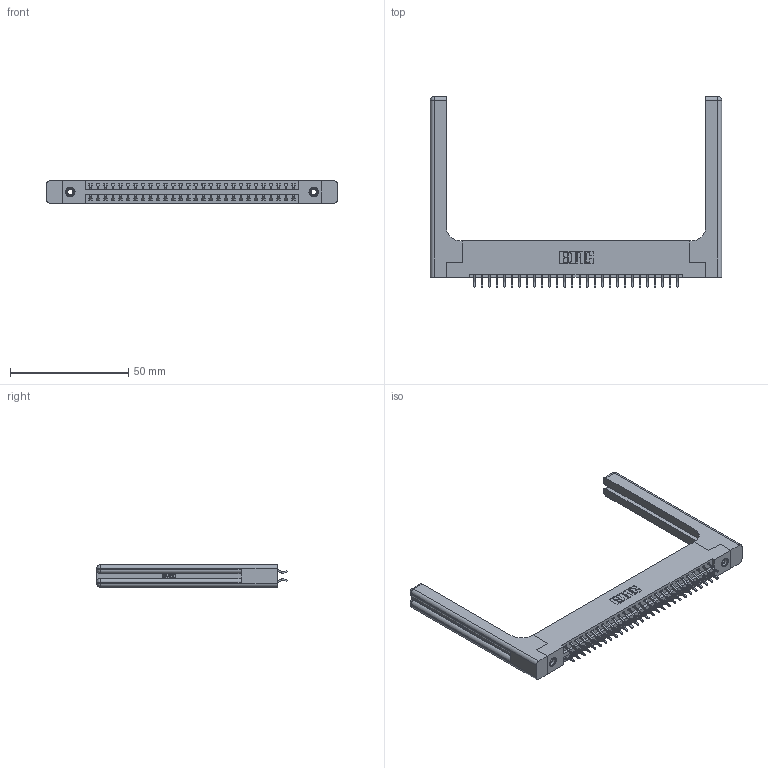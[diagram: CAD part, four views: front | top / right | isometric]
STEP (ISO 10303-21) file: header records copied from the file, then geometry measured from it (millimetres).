
FILE_DESCRIPTION (( 'STEP AP203' ), '1' );
FILE_NAME ('396-056-556-258.STEP', '2019-10-30T15:51:50', ( '' ), ( '' ), 'SwSTEP 2.0', 'SolidWorks 2016', '' );
FILE_SCHEMA (( 'CONFIG_CONTROL_DESIGN' ));
Length unit declared in the file: inch
Products named in the file (5): 345-250-001_345-250-001-102; 346 Part_Flush Mounting Lugs - 0.156 Dia-TH; 345-292-001_556 Tail; 346-220-058_345-220-058; 396-056-556-258
Assembly tree (61 placements, depth 2):
  396-056-556-258
    346 Part_Flush Mounting Lugs - 0.156 Dia-TH
    345-292-001_556 Tail  x56
    345-250-001_345-250-001-102  x2
    346-220-058_345-220-058  x2
Bounding box: 122.96 x 80.53 x 9.4 mm (x, y, z)
Volume: 19373.6 mm3; surface area: 21029.6 mm2
Topology: 61 solids, 61 shells, 3626 faces, 10683 edges, 7026 vertices
Faces by surface type: plane 2408, cylinder 1158, bspline 36, cone 12, sphere 8, torus 4
Entity records: 25560 total; most frequent: CARTESIAN_POINT 5253, ORIENTED_EDGE 3972, DIRECTION 3602, EDGE_CURVE 1986, LINE 1642, VECTOR 1642, VERTEX_POINT 1314, AXIS2_PLACEMENT_3D 980
